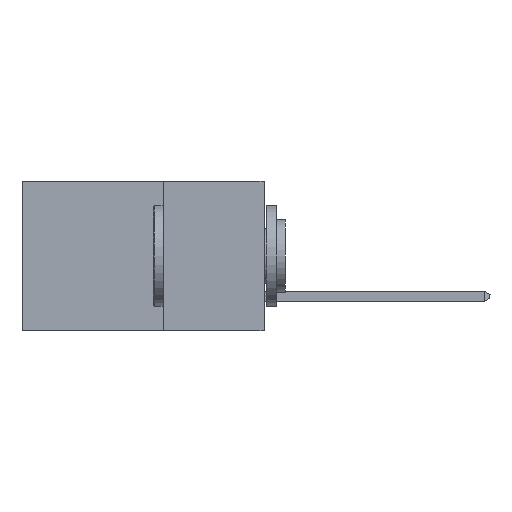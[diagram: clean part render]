
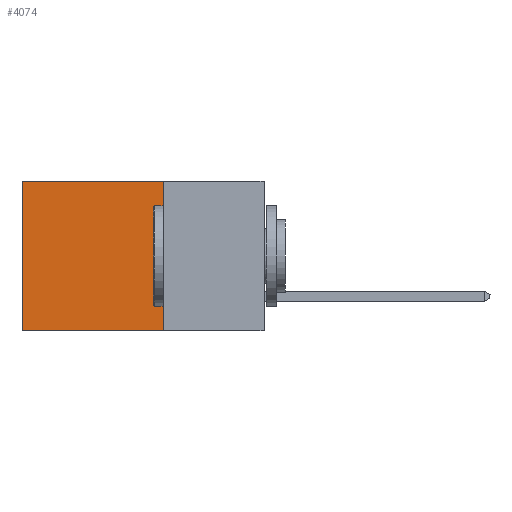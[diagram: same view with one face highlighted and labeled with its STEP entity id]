
A CAD part, left-side view. The second image highlights one B-rep face of the part: STEP entity #4074.
In plain terms, the highlighted planar face has unit normal (-1, 0, 0).
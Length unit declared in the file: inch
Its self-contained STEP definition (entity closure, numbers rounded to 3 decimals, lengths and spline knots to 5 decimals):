
#952 = LINE ( 'NONE', #10778, #11934 ) ;
#3030 = LINE ( 'NONE', #16607, #26569 ) ;
#3517 = VERTEX_POINT ( 'NONE', #11101 ) ;
#3714 = EDGE_CURVE ( 'NONE', #22791, #11437, #6764, .T. ) ;
#4074 = ADVANCED_FACE ( 'NONE', ( #13467 ), #20610, .F. ) ;
#4785 = CARTESIAN_POINT ( 'NONE',  ( 0.298, 0.6, -0.37 ) ) ;
#6764 = LINE ( 'NONE', #26392, #19362 ) ;
#7228 = ORIENTED_EDGE ( 'NONE', *, *, #3714, .T. ) ;
#8622 = LINE ( 'NONE', #24621, #15746 ) ;
#9401 = DIRECTION ( 'NONE',  ( 0., 0., -1. ) ) ;
#10778 = CARTESIAN_POINT ( 'NONE',  ( 0.298, 0.25, 0. ) ) ;
#10850 = EDGE_CURVE ( 'NONE', #3517, #11437, #8622, .T. ) ;
#11101 = CARTESIAN_POINT ( 'NONE',  ( 0.298, 0.25, -0.37 ) ) ;
#11437 = VERTEX_POINT ( 'NONE', #4785 ) ;
#11934 = VECTOR ( 'NONE', #28299, 39.37008 ) ;
#12110 = AXIS2_PLACEMENT_3D ( 'NONE', #28689, #29542, #9401 ) ;
#12362 = CARTESIAN_POINT ( 'NONE',  ( 0.298, 0.25, 0. ) ) ;
#12474 = ORIENTED_EDGE ( 'NONE', *, *, #25597, .F. ) ;
#13467 = FACE_OUTER_BOUND ( 'NONE', #28502, .T. ) ;
#13972 = DIRECTION ( 'NONE',  ( 0., 0., -1. ) ) ;
#13999 = DIRECTION ( 'NONE',  ( 0., 0., -1. ) ) ;
#15746 = VECTOR ( 'NONE', #17166, 39.37008 ) ;
#16607 = CARTESIAN_POINT ( 'NONE',  ( 0.298, 0.25, 0. ) ) ;
#17166 = DIRECTION ( 'NONE',  ( 0., 1., 0. ) ) ;
#17521 = ORIENTED_EDGE ( 'NONE', *, *, #10850, .F. ) ;
#19362 = VECTOR ( 'NONE', #13999, 39.37008 ) ;
#20334 = VERTEX_POINT ( 'NONE', #12362 ) ;
#20610 = PLANE ( 'NONE',  #12110 ) ;
#22349 = ORIENTED_EDGE ( 'NONE', *, *, #30297, .T. ) ;
#22791 = VERTEX_POINT ( 'NONE', #30570 ) ;
#24621 = CARTESIAN_POINT ( 'NONE',  ( 0.298, 0.25, -0.37 ) ) ;
#25597 = EDGE_CURVE ( 'NONE', #20334, #3517, #3030, .T. ) ;
#26392 = CARTESIAN_POINT ( 'NONE',  ( 0.298, 0.6, 0. ) ) ;
#26569 = VECTOR ( 'NONE', #13972, 39.37008 ) ;
#28299 = DIRECTION ( 'NONE',  ( 0., 1., 0. ) ) ;
#28502 = EDGE_LOOP ( 'NONE', ( #7228, #17521, #12474, #22349 ) ) ;
#28689 = CARTESIAN_POINT ( 'NONE',  ( 0.298, 0.25, 0. ) ) ;
#29542 = DIRECTION ( 'NONE',  ( 1., 0., 0. ) ) ;
#30297 = EDGE_CURVE ( 'NONE', #20334, #22791, #952, .T. ) ;
#30570 = CARTESIAN_POINT ( 'NONE',  ( 0.298, 0.6, 0. ) ) ;
